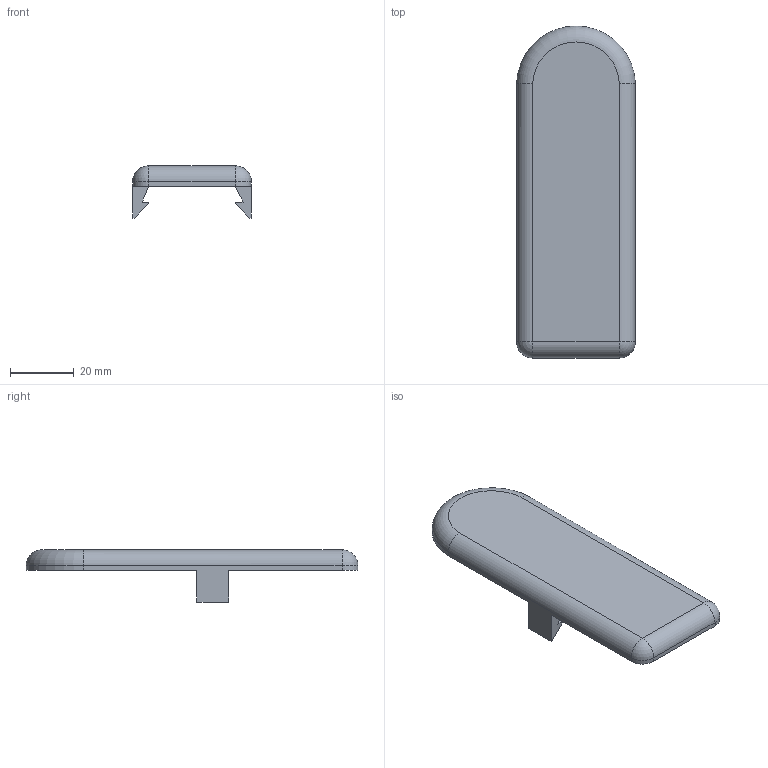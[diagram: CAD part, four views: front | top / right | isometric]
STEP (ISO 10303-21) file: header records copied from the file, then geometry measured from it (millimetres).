
FILE_DESCRIPTION (( 'STEP AP214' ), '1' );
FILE_NAME ('1-4_Inch_Buttpad_Extension.step', '2014-05-14T06:09:02', ( 'WarFairy' ), ( '' ), 'SwSTEP 2.0', 'SolidWorks 2013', '' );
FILE_SCHEMA (( 'AUTOMOTIVE_DESIGN' ));
Length unit declared in the file: inch
Products named in the file (1): 1-4_Inch_Buttpad_Extension
Bounding box: 37.13 x 103.84 x 16.35 mm (x, y, z)
Volume: 20126.1 mm3; surface area: 9710.2 mm2
Topology: 1 solids, 1 shells, 44 faces, 110 edges, 68 vertices
Faces by surface type: plane 34, cylinder 7, sphere 2, torus 1
Entity records: 1349 total; most frequent: CARTESIAN_POINT 265, ORIENTED_EDGE 216, DIRECTION 209, EDGE_CURVE 108, LINE 93, VECTOR 93, VERTEX_POINT 68, AXIS2_PLACEMENT_3D 58
